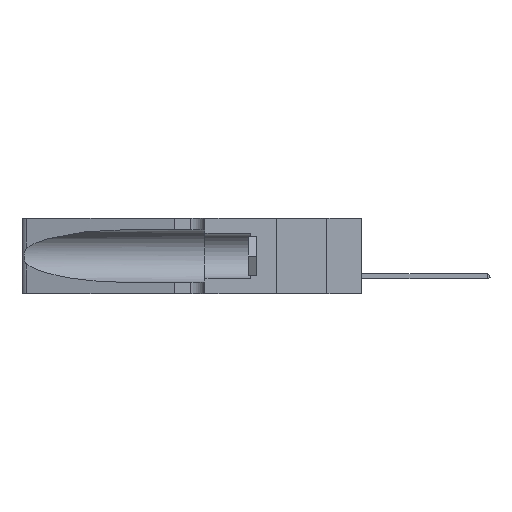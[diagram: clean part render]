
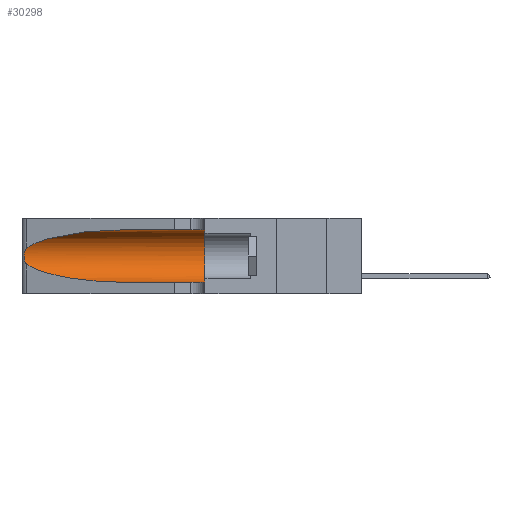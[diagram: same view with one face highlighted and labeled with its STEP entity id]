
A CAD part, left-side view. The second image highlights one B-rep face of the part: STEP entity #30298.
In plain terms, the highlighted cylindrical face has radius 3.308 mm (diameter 6.617 mm), a partial arc.
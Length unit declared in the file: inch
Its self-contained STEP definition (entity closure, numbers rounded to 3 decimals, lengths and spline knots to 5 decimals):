
#24 = CARTESIAN_POINT ( 'NONE',  ( 0.25487, 1.22718, 0.14631 ) ) ;
#858 = CARTESIAN_POINT ( 'NONE',  ( 0.1305, 0.35, 0.185 ) ) ;
#1547 = CARTESIAN_POINT ( 'NONE',  ( 0.25555, 1.22994, 0.2215 ) ) ;
#1637 = B_SPLINE_CURVE_WITH_KNOTS ( 'NONE', 3,
 ( #1782, #1547, #28101, #4407, #25478, #22833, #27866, #7131, #12066, #9792, #20204, #6787, #19852, #9325 ),
 .UNSPECIFIED., .F., .F.,
 ( 4, 2, 2, 2, 2, 2, 4 ),
 ( 0., 0.00027, 0.00053, 0.00107, 0.0016, 0.00187, 0.00214 ),
 .UNSPECIFIED. ) ;
#1782 = CARTESIAN_POINT ( 'NONE',  ( 0.25487, 1.22718, 0.22369 ) ) ;
#1881 = DIRECTION ( 'NONE',  ( 0., -1., 0. ) ) ;
#1980 = VERTEX_POINT ( 'NONE', #33504 ) ;
#2885 = CARTESIAN_POINT ( 'NONE',  ( 0.25487, 1.22718, 0.14631 ) ) ;
#3770 = LINE ( 'NONE', #18001, #18891 ) ;
#4003 = ORIENTED_EDGE ( 'NONE', *, *, #19786, .T. ) ;
#4407 = CARTESIAN_POINT ( 'NONE',  ( 0.25787, 1.23484, 0.2124 ) ) ;
#4961 = EDGE_LOOP ( 'NONE', ( #31771, #18122, #4003, #7776, #13309, #9172 ) ) ;
#5631 = EDGE_CURVE ( 'NONE', #13005, #9273, #14491, .T. ) ;
#5698 = EDGE_CURVE ( 'NONE', #1980, #5845, #17242, .T. ) ;
#5764 = LINE ( 'NONE', #16251, #32822 ) ;
#5845 = VERTEX_POINT ( 'NONE', #24805 ) ;
#6127 = CARTESIAN_POINT ( 'NONE',  ( 0.1305, 0.72297, 0.31525 ) ) ;
#6787 = CARTESIAN_POINT ( 'NONE',  ( 0.25639, 1.23186, 0.15144 ) ) ;
#7131 = CARTESIAN_POINT ( 'NONE',  ( 0.26075, 1.23896, 0.178 ) ) ;
#7776 = ORIENTED_EDGE ( 'NONE', *, *, #15251, .T. ) ;
#8118 = CARTESIAN_POINT ( 'NONE',  ( 0.1305, 1.61858, 0.185 ) ) ;
#8361 = EDGE_CURVE ( 'NONE', #13005, #1980, #3770, .T. ) ;
#8520 = CARTESIAN_POINT ( 'NONE',  ( 0.25487, 1.22718, 0.22369 ) ) ;
#8634 = FACE_OUTER_BOUND ( 'NONE', #4961, .T. ) ;
#9172 = ORIENTED_EDGE ( 'NONE', *, *, #8361, .F. ) ;
#9177 = AXIS2_PLACEMENT_3D ( 'NONE', #858, #19174, #21700 ) ;
#9273 = VERTEX_POINT ( 'NONE', #18005 ) ;
#9325 = CARTESIAN_POINT ( 'NONE',  ( 0.25487, 1.22718, 0.14631 ) ) ;
#9792 = CARTESIAN_POINT ( 'NONE',  ( 0.25856, 1.23593, 0.16098 ) ) ;
#12066 = CARTESIAN_POINT ( 'NONE',  ( 0.26017, 1.23833, 0.17102 ) ) ;
#12206 = EDGE_CURVE ( 'NONE', #9273, #22421, #1637, .T. ) ;
#12723 = CARTESIAN_POINT ( 'NONE',  ( 0.2373, 1.15595, 0.08982 ) ) ;
#12953 = CARTESIAN_POINT ( 'NONE',  ( 0.18966, 0.96281, 0.05475 ) ) ;
#13005 = VERTEX_POINT ( 'NONE', #14142 ) ;
#13309 = ORIENTED_EDGE ( 'NONE', *, *, #5698, .F. ) ;
#13377 = DIRECTION ( 'NONE',  ( 0., -1., 0. ) ) ;
#13677 = CARTESIAN_POINT ( 'NONE',  ( 0.1305, 0.72297, 0.05475 ) ) ;
#14018 = CARTESIAN_POINT ( 'NONE',  ( 0.18966, 0.96281, 0.31525 ) ) ;
#14142 = CARTESIAN_POINT ( 'NONE',  ( 0.1305, 0.72297, 0.31525 ) ) ;
#14491 =( BOUNDED_CURVE ( )  B_SPLINE_CURVE ( 3, ( #6127, #14018, #24198, #8520 ),
 .UNSPECIFIED., .F., .F. ) 
 B_SPLINE_CURVE_WITH_KNOTS ( ( 4, 4 ),
 ( 1.5708, 2.84003 ),
 .UNSPECIFIED. ) 
 CURVE ( )  GEOMETRIC_REPRESENTATION_ITEM ( )  RATIONAL_B_SPLINE_CURVE ( ( 1., 0.87, 0.87, 1. ) ) 
 REPRESENTATION_ITEM ( '' )  );
#15251 = EDGE_CURVE ( 'NONE', #31124, #5845, #5764, .T. ) ;
#16251 = CARTESIAN_POINT ( 'NONE',  ( 0.1305, 1.61858, 0.05475 ) ) ;
#17242 = CIRCLE ( 'NONE', #9177, 0.13025 ) ;
#17628 = AXIS2_PLACEMENT_3D ( 'NONE', #8118, #31736, #21288 ) ;
#18001 = CARTESIAN_POINT ( 'NONE',  ( 0.1305, 1.61858, 0.31525 ) ) ;
#18005 = CARTESIAN_POINT ( 'NONE',  ( 0.25487, 1.22718, 0.22369 ) ) ;
#18122 = ORIENTED_EDGE ( 'NONE', *, *, #12206, .T. ) ;
#18891 = VECTOR ( 'NONE', #1881, 39.37008 ) ;
#19174 = DIRECTION ( 'NONE',  ( 0., 1., 0. ) ) ;
#19786 = EDGE_CURVE ( 'NONE', #22421, #31124, #21349, .T. ) ;
#19852 = CARTESIAN_POINT ( 'NONE',  ( 0.25555, 1.22993, 0.14849 ) ) ;
#20204 = CARTESIAN_POINT ( 'NONE',  ( 0.25789, 1.23486, 0.15765 ) ) ;
#21288 = DIRECTION ( 'NONE',  ( 0., 0., -1. ) ) ;
#21349 =( BOUNDED_CURVE ( )  B_SPLINE_CURVE ( 3, ( #24, #12723, #12953, #26227 ),
 .UNSPECIFIED., .F., .F. ) 
 B_SPLINE_CURVE_WITH_KNOTS ( ( 4, 4 ),
 ( 3.44316, 4.71239 ),
 .UNSPECIFIED. ) 
 CURVE ( )  GEOMETRIC_REPRESENTATION_ITEM ( )  RATIONAL_B_SPLINE_CURVE ( ( 1., 0.87, 0.87, 1. ) ) 
 REPRESENTATION_ITEM ( '' )  );
#21700 = DIRECTION ( 'NONE',  ( 0., 0., 1. ) ) ;
#22162 = CYLINDRICAL_SURFACE ( 'NONE', #17628, 0.13025 ) ;
#22421 = VERTEX_POINT ( 'NONE', #2885 ) ;
#22833 = CARTESIAN_POINT ( 'NONE',  ( 0.26018, 1.23835, 0.19895 ) ) ;
#24198 = CARTESIAN_POINT ( 'NONE',  ( 0.2373, 1.15595, 0.28018 ) ) ;
#24805 = CARTESIAN_POINT ( 'NONE',  ( 0.1305, 0.35, 0.05475 ) ) ;
#25478 = CARTESIAN_POINT ( 'NONE',  ( 0.25854, 1.2359, 0.20912 ) ) ;
#26227 = CARTESIAN_POINT ( 'NONE',  ( 0.1305, 0.72297, 0.05475 ) ) ;
#27866 = CARTESIAN_POINT ( 'NONE',  ( 0.26075, 1.23896, 0.19203 ) ) ;
#28101 = CARTESIAN_POINT ( 'NONE',  ( 0.25639, 1.23184, 0.21858 ) ) ;
#30298 = ADVANCED_FACE ( 'NONE', ( #8634 ), #22162, .F. ) ;
#31124 = VERTEX_POINT ( 'NONE', #13677 ) ;
#31736 = DIRECTION ( 'NONE',  ( 0., -1., 0. ) ) ;
#31771 = ORIENTED_EDGE ( 'NONE', *, *, #5631, .T. ) ;
#32822 = VECTOR ( 'NONE', #13377, 39.37008 ) ;
#33504 = CARTESIAN_POINT ( 'NONE',  ( 0.1305, 0.35, 0.31525 ) ) ;
